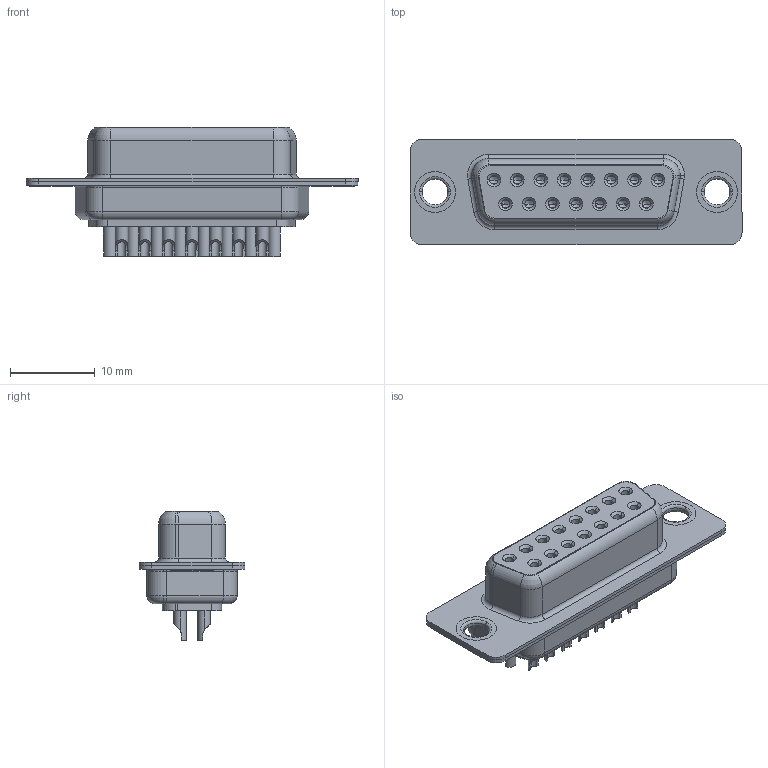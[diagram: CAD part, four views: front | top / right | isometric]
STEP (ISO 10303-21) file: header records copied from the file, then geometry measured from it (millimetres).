
FILE_DESCRIPTION (( 'STEP AP203' ), '1' );
FILE_NAME ('628-M15-222-LN1.STEP', '2021-04-26T13:51:26', ( '' ), ( '' ), 'SwSTEP 2.0', 'SolidWorks 2020', '' );
FILE_SCHEMA (( 'CONFIG_CONTROL_DESIGN' ));
Length unit declared in the file: millimetre
Products named in the file (7): 628M Contact Row 2_22; 628M Shell Front_15 Contacts; 628-M15-222-LN1; 628M Contact Row 1_22; 628M Housing_15 Contacts; 628M Shell Rear_15 Contacts; 628M Thru Hole Rivet
Assembly tree (20 placements, depth 2):
  628-M15-222-LN1
    628M Housing_15 Contacts
    628M Shell Front_15 Contacts
    628M Shell Rear_15 Contacts
    628M Contact Row 1_22  x8
    628M Contact Row 2_22  x7
    628M Thru Hole Rivet  x2
Bounding box: 39.2 x 12.5 x 15.25 mm (x, y, z)
Volume: 2414.6 mm3; surface area: 6178.6 mm2
Topology: 20 solids, 20 shells, 1079 faces, 2643 edges, 1631 vertices
Faces by surface type: cylinder 436, plane 323, torus 185, cone 135
Entity records: 16128 total; most frequent: DIRECTION 2853, CARTESIAN_POINT 2722, ORIENTED_EDGE 2382, AXIS2_PLACEMENT_3D 1192, EDGE_CURVE 1191, VERTEX_POINT 749, CIRCLE 656, EDGE_LOOP 616
